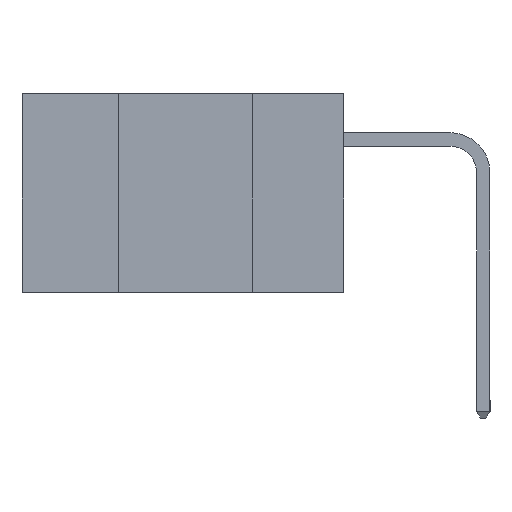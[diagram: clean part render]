
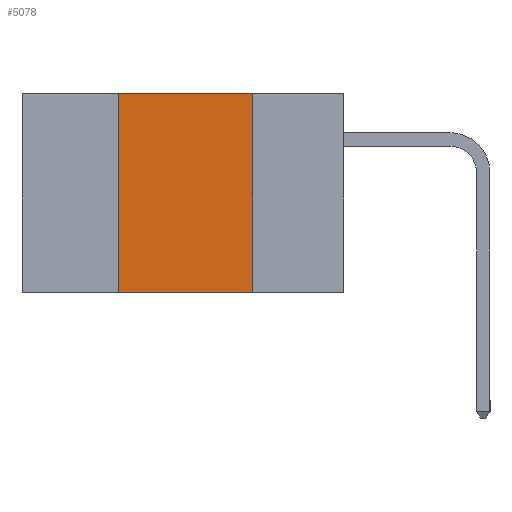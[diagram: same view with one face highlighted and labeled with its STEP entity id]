
A CAD part, left-side view. The second image highlights one B-rep face of the part: STEP entity #5078.
In plain terms, the highlighted planar face has unit normal (-1, 0, 0).
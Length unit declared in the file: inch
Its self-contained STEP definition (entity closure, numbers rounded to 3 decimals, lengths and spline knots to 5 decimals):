
#242 = VERTEX_POINT ( 'NONE', #6466 ) ;
#429 = DIRECTION ( 'NONE',  ( 0., 0., -1. ) ) ;
#445 = CARTESIAN_POINT ( 'NONE',  ( 0., 0.6, 0. ) ) ;
#464 = DIRECTION ( 'NONE',  ( 1., 0., 0. ) ) ;
#502 = PLANE ( 'NONE',  #9490 ) ;
#1261 = CARTESIAN_POINT ( 'NONE',  ( 0., 0.17, 0. ) ) ;
#1498 = CARTESIAN_POINT ( 'NONE',  ( 0., 0.6, 0. ) ) ;
#1731 = VECTOR ( 'NONE', #8528, 39.37008 ) ;
#1842 = ORIENTED_EDGE ( 'NONE', *, *, #7466, .F. ) ;
#1996 = CARTESIAN_POINT ( 'NONE',  ( 0., 0.17, -0.37 ) ) ;
#3156 = CARTESIAN_POINT ( 'NONE',  ( 0., 0.42, -0.37 ) ) ;
#4249 = EDGE_CURVE ( 'NONE', #10378, #12141, #4703, .T. ) ;
#4386 = DIRECTION ( 'NONE',  ( 0., -1., 0. ) ) ;
#4506 = CARTESIAN_POINT ( 'NONE',  ( 0., 0.6, -0.37 ) ) ;
#4703 = LINE ( 'NONE', #4506, #11770 ) ;
#4942 = LINE ( 'NONE', #445, #11718 ) ;
#4976 = FACE_OUTER_BOUND ( 'NONE', #11456, .T. ) ;
#5078 = ADVANCED_FACE ( 'NONE', ( #4976 ), #502, .F. ) ;
#5082 = CARTESIAN_POINT ( 'NONE',  ( 0., 0.42, -0.37 ) ) ;
#5274 = DIRECTION ( 'NONE',  ( 0., -1., 0. ) ) ;
#6466 = CARTESIAN_POINT ( 'NONE',  ( 0., 0.42, 0. ) ) ;
#6808 = LINE ( 'NONE', #1996, #1731 ) ;
#6925 = ORIENTED_EDGE ( 'NONE', *, *, #9708, .F. ) ;
#6968 = DIRECTION ( 'NONE',  ( 0., 0., 1. ) ) ;
#7466 = EDGE_CURVE ( 'NONE', #242, #10434, #4942, .T. ) ;
#7785 = CARTESIAN_POINT ( 'NONE',  ( 0., 0.17, -0.37 ) ) ;
#7962 = VECTOR ( 'NONE', #6968, 39.37008 ) ;
#8528 = DIRECTION ( 'NONE',  ( 0., 0., -1. ) ) ;
#9019 = ORIENTED_EDGE ( 'NONE', *, *, #10228, .F. ) ;
#9490 = AXIS2_PLACEMENT_3D ( 'NONE', #1498, #464, #429 ) ;
#9600 = ORIENTED_EDGE ( 'NONE', *, *, #4249, .T. ) ;
#9708 = EDGE_CURVE ( 'NONE', #10378, #242, #10369, .T. ) ;
#10228 = EDGE_CURVE ( 'NONE', #10434, #12141, #6808, .T. ) ;
#10369 = LINE ( 'NONE', #5082, #7962 ) ;
#10378 = VERTEX_POINT ( 'NONE', #3156 ) ;
#10434 = VERTEX_POINT ( 'NONE', #1261 ) ;
#11456 = EDGE_LOOP ( 'NONE', ( #9019, #1842, #6925, #9600 ) ) ;
#11718 = VECTOR ( 'NONE', #5274, 39.37008 ) ;
#11770 = VECTOR ( 'NONE', #4386, 39.37008 ) ;
#12141 = VERTEX_POINT ( 'NONE', #7785 ) ;
